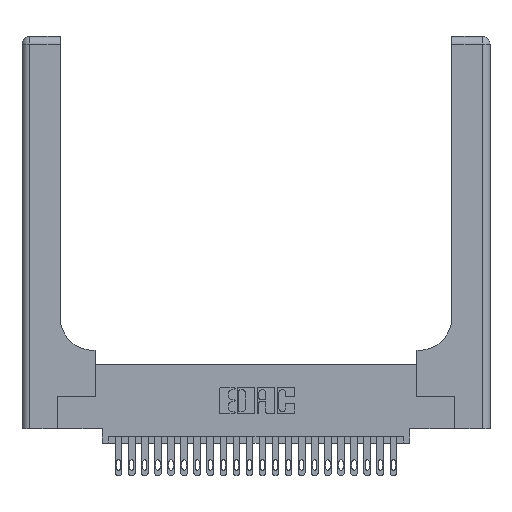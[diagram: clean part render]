
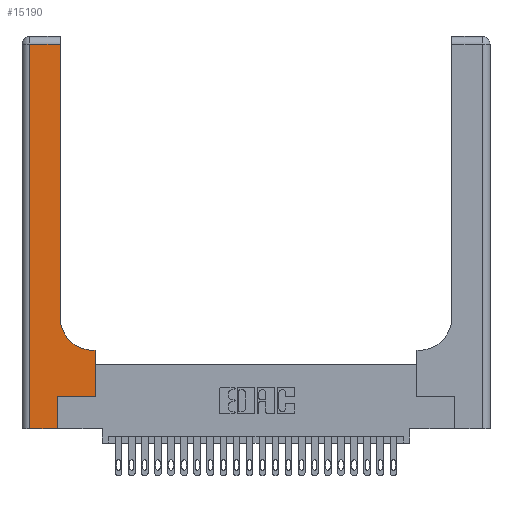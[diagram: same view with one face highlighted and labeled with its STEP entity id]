
A CAD part, top view. The second image highlights one B-rep face of the part: STEP entity #15190.
In plain terms, the highlighted planar face has unit normal (0, 0, 1).
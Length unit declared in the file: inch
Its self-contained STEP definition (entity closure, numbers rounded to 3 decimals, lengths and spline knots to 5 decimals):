
#567 = CARTESIAN_POINT ( 'NONE',  ( 0., 0., 0.37 ) ) ;
#663 = ORIENTED_EDGE ( 'NONE', *, *, #6622, .T. ) ;
#705 = EDGE_LOOP ( 'NONE', ( #663, #22838, #6604, #19833, #20894, #13202, #3582, #19327, #18973 ) ) ;
#841 = EDGE_CURVE ( 'NONE', #24578, #7211, #18652, .T. ) ;
#925 = VERTEX_POINT ( 'NONE', #14362 ) ;
#1258 = VERTEX_POINT ( 'NONE', #19476 ) ;
#2014 = DIRECTION ( 'NONE',  ( 0., 1., 0. ) ) ;
#2039 = DIRECTION ( 'NONE',  ( 0., 0., -1. ) ) ;
#2094 = EDGE_CURVE ( 'NONE', #7211, #17456, #15221, .T. ) ;
#2217 = CARTESIAN_POINT ( 'NONE',  ( 0., 3., 0.37 ) ) ;
#2908 = CARTESIAN_POINT ( 'NONE',  ( 0.2915, 0.6, 0.37 ) ) ;
#3582 = ORIENTED_EDGE ( 'NONE', *, *, #4614, .T. ) ;
#4614 = EDGE_CURVE ( 'NONE', #12880, #925, #13272, .T. ) ;
#4728 = AXIS2_PLACEMENT_3D ( 'NONE', #2217, #2039, #21476 ) ;
#4875 = DIRECTION ( 'NONE',  ( -1., 0., 0. ) ) ;
#4985 = DIRECTION ( 'NONE',  ( 0., 1., 0. ) ) ;
#5043 = VERTEX_POINT ( 'NONE', #16535 ) ;
#5423 = VECTOR ( 'NONE', #4985, 39.37008 ) ;
#5793 = AXIS2_PLACEMENT_3D ( 'NONE', #20626, #24428, #12598 ) ;
#6056 = DIRECTION ( 'NONE',  ( -1., 0., 0. ) ) ;
#6266 = VECTOR ( 'NONE', #24966, 39.37008 ) ;
#6604 = ORIENTED_EDGE ( 'NONE', *, *, #841, .T. ) ;
#6622 = EDGE_CURVE ( 'NONE', #19455, #5043, #10762, .T. ) ;
#6841 = CARTESIAN_POINT ( 'NONE',  ( 0.06, 3., 0.37 ) ) ;
#7211 = VERTEX_POINT ( 'NONE', #22859 ) ;
#8326 = DIRECTION ( 'NONE',  ( 1., 0., 0. ) ) ;
#9403 = CARTESIAN_POINT ( 'NONE',  ( 0.2915, 3., 0.37 ) ) ;
#9612 = LINE ( 'NONE', #2908, #16926 ) ;
#10098 = DIRECTION ( 'NONE',  ( 1., 0., 0. ) ) ;
#10410 = EDGE_CURVE ( 'NONE', #22428, #19455, #17597, .T. ) ;
#10762 = LINE ( 'NONE', #9403, #20838 ) ;
#12598 = DIRECTION ( 'NONE',  ( 1., 0., 0. ) ) ;
#12785 = LINE ( 'NONE', #24066, #14334 ) ;
#12880 = VERTEX_POINT ( 'NONE', #19254 ) ;
#13202 = ORIENTED_EDGE ( 'NONE', *, *, #20582, .T. ) ;
#13272 = LINE ( 'NONE', #21080, #6266 ) ;
#14305 = CARTESIAN_POINT ( 'NONE',  ( 0.2915, 0.85, 0.37 ) ) ;
#14334 = VECTOR ( 'NONE', #8326, 39.37008 ) ;
#14362 = CARTESIAN_POINT ( 'NONE',  ( 0.5585, 0.6, 0.37 ) ) ;
#15150 = LINE ( 'NONE', #16794, #5423 ) ;
#15190 = ADVANCED_FACE ( 'NONE', ( #15270 ), #23486, .F. ) ;
#15221 = LINE ( 'NONE', #567, #24382 ) ;
#15270 = FACE_OUTER_BOUND ( 'NONE', #705, .T. ) ;
#16000 = CARTESIAN_POINT ( 'NONE',  ( 0.5415, 0.6, 0.37 ) ) ;
#16535 = CARTESIAN_POINT ( 'NONE',  ( 0.2915, 2.94, 0.37 ) ) ;
#16794 = CARTESIAN_POINT ( 'NONE',  ( 0.269, 0., 0.37 ) ) ;
#16926 = VECTOR ( 'NONE', #4875, 39.37008 ) ;
#17111 = VECTOR ( 'NONE', #6056, 39.37008 ) ;
#17456 = VERTEX_POINT ( 'NONE', #25197 ) ;
#17597 = CIRCLE ( 'NONE', #5793, 0.25 ) ;
#17695 = EDGE_CURVE ( 'NONE', #925, #22428, #9612, .T. ) ;
#18652 = LINE ( 'NONE', #6841, #19568 ) ;
#18973 = ORIENTED_EDGE ( 'NONE', *, *, #10410, .T. ) ;
#19254 = CARTESIAN_POINT ( 'NONE',  ( 0.5585, 0.25, 0.37 ) ) ;
#19327 = ORIENTED_EDGE ( 'NONE', *, *, #17695, .T. ) ;
#19378 = EDGE_CURVE ( 'NONE', #5043, #24578, #20173, .T. ) ;
#19455 = VERTEX_POINT ( 'NONE', #14305 ) ;
#19476 = CARTESIAN_POINT ( 'NONE',  ( 0.269, 0.25, 0.37 ) ) ;
#19568 = VECTOR ( 'NONE', #22439, 39.37008 ) ;
#19833 = ORIENTED_EDGE ( 'NONE', *, *, #2094, .T. ) ;
#20173 = LINE ( 'NONE', #23576, #17111 ) ;
#20582 = EDGE_CURVE ( 'NONE', #1258, #12880, #12785, .T. ) ;
#20626 = CARTESIAN_POINT ( 'NONE',  ( 0.5415, 0.85, 0.37 ) ) ;
#20838 = VECTOR ( 'NONE', #2014, 39.37008 ) ;
#20894 = ORIENTED_EDGE ( 'NONE', *, *, #21912, .T. ) ;
#21080 = CARTESIAN_POINT ( 'NONE',  ( 0.5585, 0.25, 0.37 ) ) ;
#21476 = DIRECTION ( 'NONE',  ( -1., 0., 0. ) ) ;
#21656 = CARTESIAN_POINT ( 'NONE',  ( 0.06, 2.94, 0.37 ) ) ;
#21912 = EDGE_CURVE ( 'NONE', #17456, #1258, #15150, .T. ) ;
#22428 = VERTEX_POINT ( 'NONE', #16000 ) ;
#22439 = DIRECTION ( 'NONE',  ( 0., -1., 0. ) ) ;
#22838 = ORIENTED_EDGE ( 'NONE', *, *, #19378, .T. ) ;
#22859 = CARTESIAN_POINT ( 'NONE',  ( 0.06, 0., 0.37 ) ) ;
#23486 = PLANE ( 'NONE',  #4728 ) ;
#23576 = CARTESIAN_POINT ( 'NONE',  ( 0., 2.94, 0.37 ) ) ;
#24066 = CARTESIAN_POINT ( 'NONE',  ( 0.269, 0.25, 0.37 ) ) ;
#24382 = VECTOR ( 'NONE', #10098, 39.37008 ) ;
#24428 = DIRECTION ( 'NONE',  ( 0., 0., -1. ) ) ;
#24578 = VERTEX_POINT ( 'NONE', #21656 ) ;
#24966 = DIRECTION ( 'NONE',  ( 0., 1., 0. ) ) ;
#25197 = CARTESIAN_POINT ( 'NONE',  ( 0.269, 0., 0.37 ) ) ;
